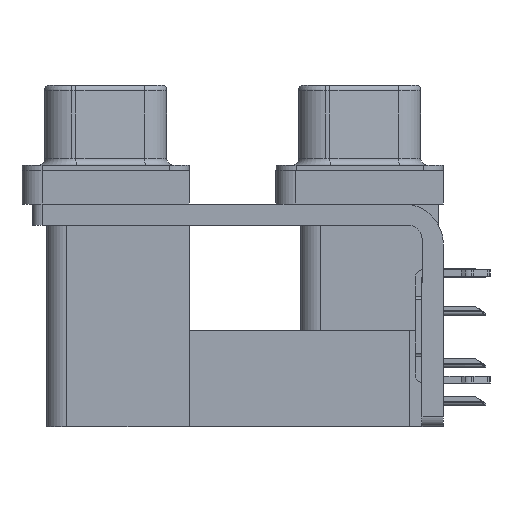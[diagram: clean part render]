
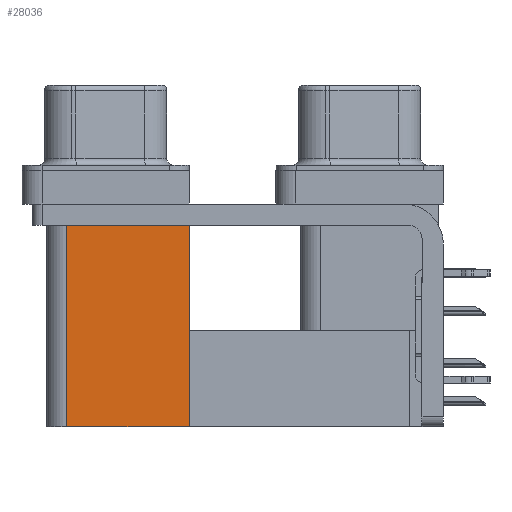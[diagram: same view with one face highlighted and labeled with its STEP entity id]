
A CAD part, left-side view. The second image highlights one B-rep face of the part: STEP entity #28036.
In plain terms, the highlighted planar face has unit normal (-1, 0, 0).
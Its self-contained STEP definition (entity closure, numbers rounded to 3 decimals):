
#249 = VERTEX_POINT ( 'NONE', #48274 ) ;
#534 = CARTESIAN_POINT ( 'NONE',  ( 3.79, 21.975, -2.5 ) ) ;
#766 = ORIENTED_EDGE ( 'NONE', *, *, #4633, .T. ) ;
#3420 = ORIENTED_EDGE ( 'NONE', *, *, #35680, .T. ) ;
#4633 = EDGE_CURVE ( 'NONE', #249, #26578, #33317, .T. ) ;
#6946 = FACE_OUTER_BOUND ( 'NONE', #8982, .T. ) ;
#7173 = DIRECTION ( 'NONE',  ( 0., 1., 0. ) ) ;
#8982 = EDGE_LOOP ( 'NONE', ( #3420, #17280, #49637, #766 ) ) ;
#12776 = AXIS2_PLACEMENT_3D ( 'NONE', #37951, #14941, #30719 ) ;
#12814 = EDGE_CURVE ( 'NONE', #249, #41529, #14669, .T. ) ;
#13829 = VECTOR ( 'NONE', #20577, 1000. ) ;
#13946 = VECTOR ( 'NONE', #17309, 1000. ) ;
#14669 = LINE ( 'NONE', #42047, #14710 ) ;
#14710 = VECTOR ( 'NONE', #7173, 1000. ) ;
#14941 = DIRECTION ( 'NONE',  ( 1., 0., 0. ) ) ;
#17280 = ORIENTED_EDGE ( 'NONE', *, *, #38566, .F. ) ;
#17309 = DIRECTION ( 'NONE',  ( 0., 0., 1. ) ) ;
#18111 = VECTOR ( 'NONE', #36490, 1000. ) ;
#20577 = DIRECTION ( 'NONE',  ( 0., 1., 0. ) ) ;
#22024 = VERTEX_POINT ( 'NONE', #534 ) ;
#22210 = PLANE ( 'NONE',  #12776 ) ;
#24530 = CARTESIAN_POINT ( 'NONE',  ( 3.79, 21.975, -19.2 ) ) ;
#26578 = VERTEX_POINT ( 'NONE', #29700 ) ;
#28036 = ADVANCED_FACE ( 'NONE', ( #6946 ), #22210, .F. ) ;
#28834 = CARTESIAN_POINT ( 'NONE',  ( 3.79, 12.775, -2.5 ) ) ;
#29700 = CARTESIAN_POINT ( 'NONE',  ( 3.79, 12.775, -2.5 ) ) ;
#30719 = DIRECTION ( 'NONE',  ( 0., 0., -1. ) ) ;
#33317 = LINE ( 'NONE', #36942, #13946 ) ;
#35680 = EDGE_CURVE ( 'NONE', #26578, #22024, #40198, .T. ) ;
#35991 = CARTESIAN_POINT ( 'NONE',  ( 3.79, 21.975, -19.2 ) ) ;
#36490 = DIRECTION ( 'NONE',  ( 0., 0., 1. ) ) ;
#36942 = CARTESIAN_POINT ( 'NONE',  ( 3.79, 12.775, -19.2 ) ) ;
#37951 = CARTESIAN_POINT ( 'NONE',  ( 3.79, 12.775, -19.2 ) ) ;
#38566 = EDGE_CURVE ( 'NONE', #41529, #22024, #44491, .T. ) ;
#40198 = LINE ( 'NONE', #28834, #13829 ) ;
#41529 = VERTEX_POINT ( 'NONE', #24530 ) ;
#42047 = CARTESIAN_POINT ( 'NONE',  ( 3.79, 12.775, -19.2 ) ) ;
#44491 = LINE ( 'NONE', #35991, #18111 ) ;
#48274 = CARTESIAN_POINT ( 'NONE',  ( 3.79, 12.775, -19.2 ) ) ;
#49637 = ORIENTED_EDGE ( 'NONE', *, *, #12814, .F. ) ;
